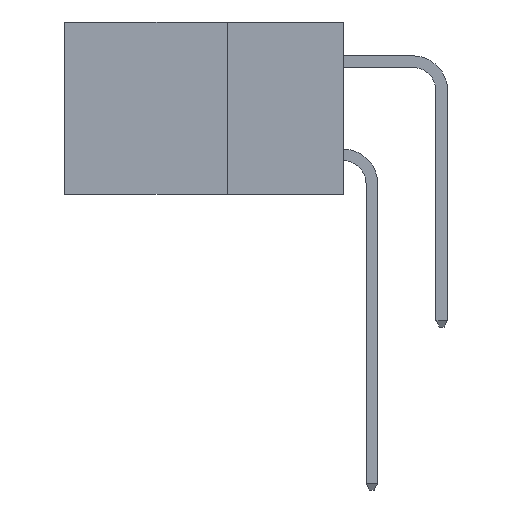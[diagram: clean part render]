
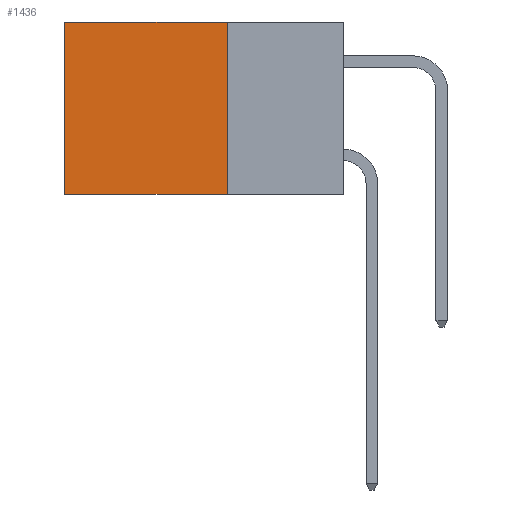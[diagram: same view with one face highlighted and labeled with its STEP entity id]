
A CAD part, left-side view. The second image highlights one B-rep face of the part: STEP entity #1436.
In plain terms, the highlighted planar face has unit normal (-1, 0, 0).
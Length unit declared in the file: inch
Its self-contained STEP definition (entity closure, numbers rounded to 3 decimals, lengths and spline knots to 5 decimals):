
#115 = EDGE_LOOP ( 'NONE', ( #6598, #839, #5128, #12647 ) ) ;
#697 = DIRECTION ( 'NONE',  ( 0., 0., -1. ) ) ;
#823 = PLANE ( 'NONE',  #10393 ) ;
#824 = EDGE_CURVE ( 'NONE', #5430, #11301, #8840, .T. ) ;
#839 = ORIENTED_EDGE ( 'NONE', *, *, #824, .F. ) ;
#1088 = LINE ( 'NONE', #8904, #12159 ) ;
#1420 = VERTEX_POINT ( 'NONE', #4015 ) ;
#1436 = ADVANCED_FACE ( 'NONE', ( #7524 ), #823, .F. ) ;
#2695 = DIRECTION ( 'NONE',  ( 0., 0., -1. ) ) ;
#3721 = DIRECTION ( 'NONE',  ( 0., 0., -1. ) ) ;
#3890 = LINE ( 'NONE', #5776, #9093 ) ;
#4015 = CARTESIAN_POINT ( 'NONE',  ( 0.2615, 0.6, 0. ) ) ;
#5090 = DIRECTION ( 'NONE',  ( 0., 1., 0. ) ) ;
#5128 = ORIENTED_EDGE ( 'NONE', *, *, #12251, .F. ) ;
#5430 = VERTEX_POINT ( 'NONE', #11953 ) ;
#5776 = CARTESIAN_POINT ( 'NONE',  ( 0.2615, 0.6, -0.37 ) ) ;
#6084 = VECTOR ( 'NONE', #5090, 39.37008 ) ;
#6157 = CARTESIAN_POINT ( 'NONE',  ( 0.2615, 0.25, 0. ) ) ;
#6598 = ORIENTED_EDGE ( 'NONE', *, *, #12254, .T. ) ;
#7340 = EDGE_CURVE ( 'NONE', #13065, #1420, #7774, .T. ) ;
#7380 = CARTESIAN_POINT ( 'NONE',  ( 0.2615, 0.6, -0.37 ) ) ;
#7524 = FACE_OUTER_BOUND ( 'NONE', #115, .T. ) ;
#7774 = LINE ( 'NONE', #9000, #12902 ) ;
#8726 = DIRECTION ( 'NONE',  ( 1., 0., 0. ) ) ;
#8840 = LINE ( 'NONE', #13394, #6084 ) ;
#8904 = CARTESIAN_POINT ( 'NONE',  ( 0.2615, 0.25, -0.37 ) ) ;
#9000 = CARTESIAN_POINT ( 'NONE',  ( 0.2615, 0.25, 0. ) ) ;
#9052 = DIRECTION ( 'NONE',  ( 0., 1., 0. ) ) ;
#9093 = VECTOR ( 'NONE', #3721, 39.37008 ) ;
#9946 = CARTESIAN_POINT ( 'NONE',  ( 0.2615, 0.25, -0.37 ) ) ;
#10393 = AXIS2_PLACEMENT_3D ( 'NONE', #9946, #8726, #697 ) ;
#11301 = VERTEX_POINT ( 'NONE', #7380 ) ;
#11953 = CARTESIAN_POINT ( 'NONE',  ( 0.2615, 0.25, -0.37 ) ) ;
#12159 = VECTOR ( 'NONE', #2695, 39.37008 ) ;
#12251 = EDGE_CURVE ( 'NONE', #13065, #5430, #1088, .T. ) ;
#12254 = EDGE_CURVE ( 'NONE', #1420, #11301, #3890, .T. ) ;
#12647 = ORIENTED_EDGE ( 'NONE', *, *, #7340, .T. ) ;
#12902 = VECTOR ( 'NONE', #9052, 39.37008 ) ;
#13065 = VERTEX_POINT ( 'NONE', #6157 ) ;
#13394 = CARTESIAN_POINT ( 'NONE',  ( 0.2615, 0.25, -0.37 ) ) ;
